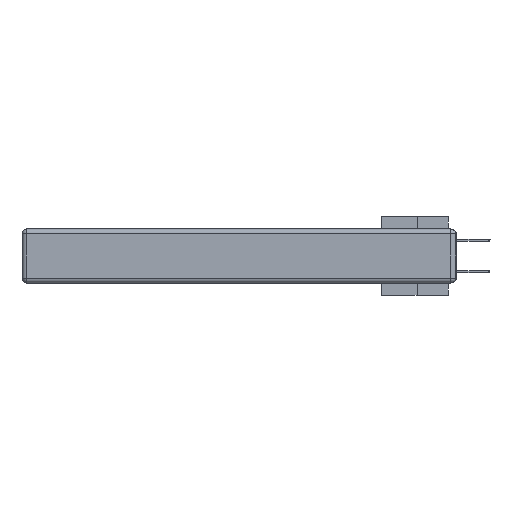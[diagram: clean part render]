
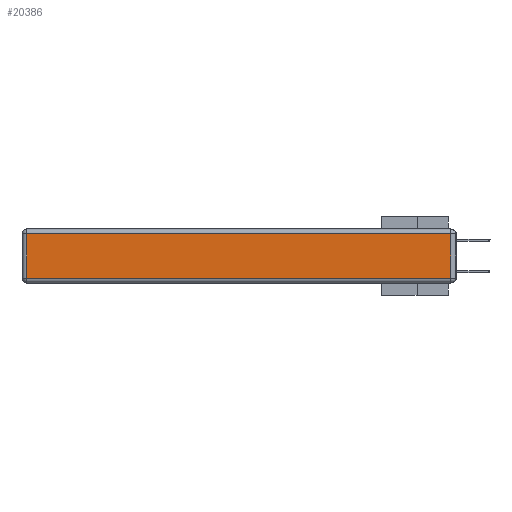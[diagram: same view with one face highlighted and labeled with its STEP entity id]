
A CAD part, left-side view. The second image highlights one B-rep face of the part: STEP entity #20386.
In plain terms, the highlighted planar face has unit normal (-1, 0, 0).
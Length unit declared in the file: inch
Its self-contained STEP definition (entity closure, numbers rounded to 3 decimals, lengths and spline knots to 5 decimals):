
#168 = VERTEX_POINT ( 'NONE', #35628 ) ;
#415 = ORIENTED_EDGE ( 'NONE', *, *, #818, .T. ) ;
#818 = EDGE_CURVE ( 'NONE', #168, #12731, #16400, .T. ) ;
#1586 = FACE_OUTER_BOUND ( 'NONE', #3800, .T. ) ;
#1890 = DIRECTION ( 'NONE',  ( 0., -1., 0. ) ) ;
#2722 = VECTOR ( 'NONE', #1890, 39.37008 ) ;
#3800 = EDGE_LOOP ( 'NONE', ( #33315, #18369, #35014, #415 ) ) ;
#4422 = PLANE ( 'NONE',  #24172 ) ;
#6639 = DIRECTION ( 'NONE',  ( 0., 0., -1. ) ) ;
#7366 = CARTESIAN_POINT ( 'NONE',  ( 0., 0.03, -0.343 ) ) ;
#7440 = CARTESIAN_POINT ( 'NONE',  ( 0., 0., -0.343 ) ) ;
#7705 = DIRECTION ( 'NONE',  ( 0., 0., 1. ) ) ;
#8710 = EDGE_CURVE ( 'NONE', #12731, #9395, #19481, .T. ) ;
#9395 = VERTEX_POINT ( 'NONE', #28622 ) ;
#9609 = CARTESIAN_POINT ( 'NONE',  ( 0., 0., -0.313 ) ) ;
#12313 = EDGE_CURVE ( 'NONE', #23320, #168, #17520, .T. ) ;
#12731 = VERTEX_POINT ( 'NONE', #24925 ) ;
#16400 = LINE ( 'NONE', #35292, #40597 ) ;
#16624 = DIRECTION ( 'NONE',  ( 0., 1., 0. ) ) ;
#17520 = LINE ( 'NONE', #35570, #21039 ) ;
#18369 = ORIENTED_EDGE ( 'NONE', *, *, #30567, .T. ) ;
#19481 = LINE ( 'NONE', #9609, #2722 ) ;
#20386 = ADVANCED_FACE ( 'NONE', ( #1586 ), #4422, .T. ) ;
#20576 = CARTESIAN_POINT ( 'NONE',  ( 0., 0.03, -0.03 ) ) ;
#21039 = VECTOR ( 'NONE', #16624, 39.37008 ) ;
#23320 = VERTEX_POINT ( 'NONE', #20576 ) ;
#24172 = AXIS2_PLACEMENT_3D ( 'NONE', #7440, #29462, #7705 ) ;
#24925 = CARTESIAN_POINT ( 'NONE',  ( 0., 2.72, -0.313 ) ) ;
#27004 = VECTOR ( 'NONE', #35459, 39.37008 ) ;
#28622 = CARTESIAN_POINT ( 'NONE',  ( 0., 0.03, -0.313 ) ) ;
#29462 = DIRECTION ( 'NONE',  ( -1., 0., 0. ) ) ;
#30567 = EDGE_CURVE ( 'NONE', #9395, #23320, #31940, .T. ) ;
#31940 = LINE ( 'NONE', #7366, #27004 ) ;
#33315 = ORIENTED_EDGE ( 'NONE', *, *, #8710, .T. ) ;
#35014 = ORIENTED_EDGE ( 'NONE', *, *, #12313, .T. ) ;
#35292 = CARTESIAN_POINT ( 'NONE',  ( 0., 2.72, -0.343 ) ) ;
#35459 = DIRECTION ( 'NONE',  ( 0., 0., 1. ) ) ;
#35570 = CARTESIAN_POINT ( 'NONE',  ( 0., 2.75, -0.03 ) ) ;
#35628 = CARTESIAN_POINT ( 'NONE',  ( 0., 2.72, -0.03 ) ) ;
#40597 = VECTOR ( 'NONE', #6639, 39.37008 ) ;
